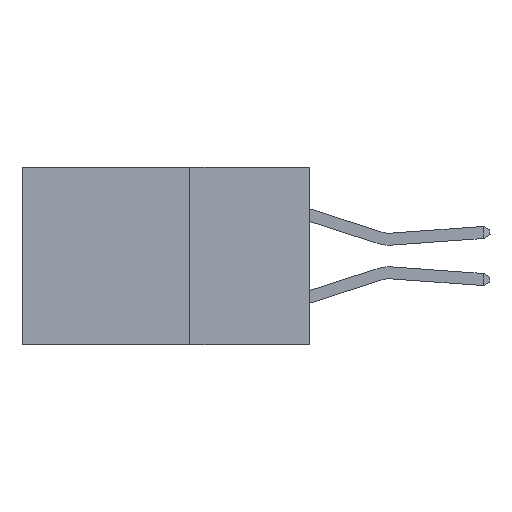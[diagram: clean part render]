
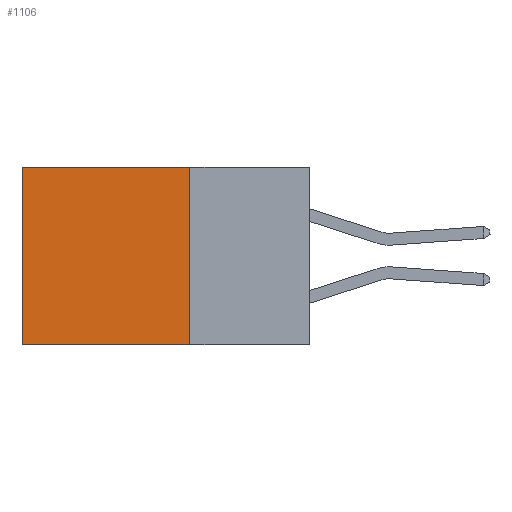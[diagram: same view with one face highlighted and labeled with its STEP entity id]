
A CAD part, left-side view. The second image highlights one B-rep face of the part: STEP entity #1106.
In plain terms, the highlighted planar face has unit normal (-1, 0, 0).
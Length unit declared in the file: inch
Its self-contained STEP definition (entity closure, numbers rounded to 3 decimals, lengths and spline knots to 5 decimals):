
#42 = DIRECTION ( 'NONE',  ( 0., 0., -1. ) ) ;
#268 = VECTOR ( 'NONE', #7765, 39.37008 ) ;
#319 = ORIENTED_EDGE ( 'NONE', *, *, #7415, .F. ) ;
#1076 = EDGE_CURVE ( 'NONE', #8014, #5834, #5276, .T. ) ;
#1106 = ADVANCED_FACE ( 'NONE', ( #6743 ), #2825, .F. ) ;
#1791 = LINE ( 'NONE', #7059, #4711 ) ;
#2375 = CARTESIAN_POINT ( 'NONE',  ( 0.2615, 0.25, -0.37 ) ) ;
#2421 = EDGE_CURVE ( 'NONE', #3862, #2526, #3642, .T. ) ;
#2460 = CARTESIAN_POINT ( 'NONE',  ( 0.2615, 0.6, -0.37 ) ) ;
#2526 = VERTEX_POINT ( 'NONE', #2375 ) ;
#2720 = CARTESIAN_POINT ( 'NONE',  ( 0.2615, 0.25, -0.37 ) ) ;
#2748 = EDGE_CURVE ( 'NONE', #3862, #8014, #1791, .T. ) ;
#2825 = PLANE ( 'NONE',  #8576 ) ;
#3014 = DIRECTION ( 'NONE',  ( 1., 0., 0. ) ) ;
#3145 = CARTESIAN_POINT ( 'NONE',  ( 0.2615, 0.25, 0. ) ) ;
#3642 = LINE ( 'NONE', #2720, #5180 ) ;
#3862 = VERTEX_POINT ( 'NONE', #3145 ) ;
#3993 = ORIENTED_EDGE ( 'NONE', *, *, #2748, .T. ) ;
#4446 = CARTESIAN_POINT ( 'NONE',  ( 0.2615, 0.25, -0.37 ) ) ;
#4711 = VECTOR ( 'NONE', #8374, 39.37008 ) ;
#5180 = VECTOR ( 'NONE', #5766, 39.37008 ) ;
#5276 = LINE ( 'NONE', #5962, #9181 ) ;
#5673 = ORIENTED_EDGE ( 'NONE', *, *, #1076, .T. ) ;
#5766 = DIRECTION ( 'NONE',  ( 0., 0., -1. ) ) ;
#5834 = VERTEX_POINT ( 'NONE', #2460 ) ;
#5962 = CARTESIAN_POINT ( 'NONE',  ( 0.2615, 0.6, -0.37 ) ) ;
#6696 = DIRECTION ( 'NONE',  ( 0., 0., -1. ) ) ;
#6743 = FACE_OUTER_BOUND ( 'NONE', #7670, .T. ) ;
#6987 = LINE ( 'NONE', #9224, #268 ) ;
#7059 = CARTESIAN_POINT ( 'NONE',  ( 0.2615, 0.25, 0. ) ) ;
#7415 = EDGE_CURVE ( 'NONE', #2526, #5834, #6987, .T. ) ;
#7670 = EDGE_LOOP ( 'NONE', ( #5673, #319, #8433, #3993 ) ) ;
#7765 = DIRECTION ( 'NONE',  ( 0., 1., 0. ) ) ;
#8014 = VERTEX_POINT ( 'NONE', #8054 ) ;
#8054 = CARTESIAN_POINT ( 'NONE',  ( 0.2615, 0.6, 0. ) ) ;
#8374 = DIRECTION ( 'NONE',  ( 0., 1., 0. ) ) ;
#8433 = ORIENTED_EDGE ( 'NONE', *, *, #2421, .F. ) ;
#8576 = AXIS2_PLACEMENT_3D ( 'NONE', #4446, #3014, #42 ) ;
#9181 = VECTOR ( 'NONE', #6696, 39.37008 ) ;
#9224 = CARTESIAN_POINT ( 'NONE',  ( 0.2615, 0.25, -0.37 ) ) ;
